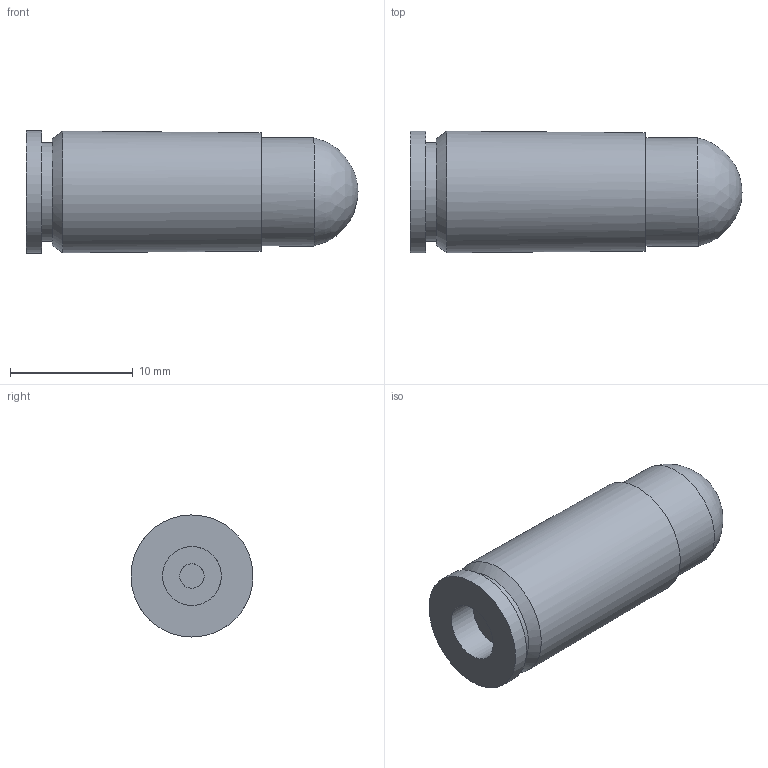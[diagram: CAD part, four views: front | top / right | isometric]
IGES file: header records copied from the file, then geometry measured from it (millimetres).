
Global section: file name: simunition 9mm v002; native system: Autodesk Inventor 2017; preprocessor: unknown; author: user; date: 20201009.140751; units: millimetre
Bounding box: 27.08 x 9.95 x 9.96 mm (x, y, z)
Volume: 1391.1 mm3; surface area: 2385.8 mm2
Topology: 4 solids, 4 shells, 61 faces, 186 edges, 132 vertices
Faces by surface type: bspline 61
